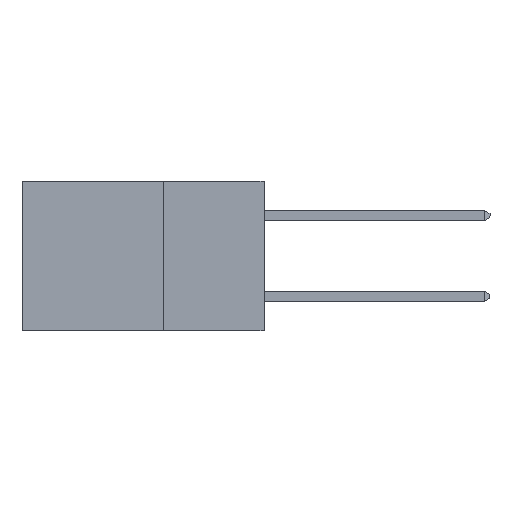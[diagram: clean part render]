
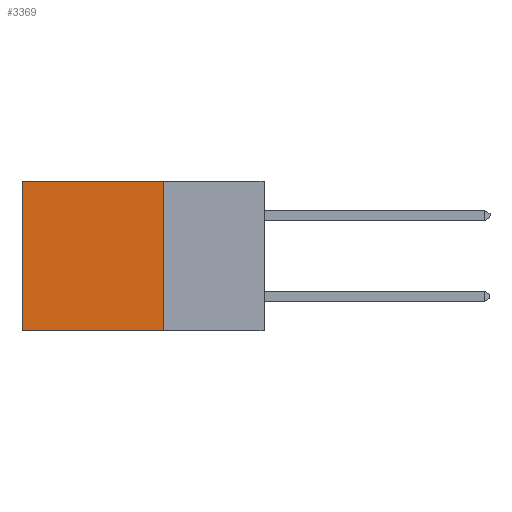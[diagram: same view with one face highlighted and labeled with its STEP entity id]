
A CAD part, left-side view. The second image highlights one B-rep face of the part: STEP entity #3369.
In plain terms, the highlighted planar face has unit normal (-1, 0, 0).
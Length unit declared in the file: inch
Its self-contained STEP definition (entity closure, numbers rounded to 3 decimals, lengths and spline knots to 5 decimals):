
#329 = PLANE ( 'NONE',  #11443 ) ;
#387 = LINE ( 'NONE', #11750, #2366 ) ;
#656 = VERTEX_POINT ( 'NONE', #1639 ) ;
#1639 = CARTESIAN_POINT ( 'NONE',  ( 0.298, 0.6, 0. ) ) ;
#1813 = DIRECTION ( 'NONE',  ( 0., 0., -1. ) ) ;
#2072 = ORIENTED_EDGE ( 'NONE', *, *, #6929, .T. ) ;
#2182 = ORIENTED_EDGE ( 'NONE', *, *, #3774, .F. ) ;
#2245 = VERTEX_POINT ( 'NONE', #4209 ) ;
#2325 = ORIENTED_EDGE ( 'NONE', *, *, #8236, .F. ) ;
#2366 = VECTOR ( 'NONE', #5428, 39.37008 ) ;
#2414 = ORIENTED_EDGE ( 'NONE', *, *, #11624, .T. ) ;
#3369 = ADVANCED_FACE ( 'NONE', ( #8489 ), #329, .F. ) ;
#3519 = DIRECTION ( 'NONE',  ( 1., 0., 0. ) ) ;
#3774 = EDGE_CURVE ( 'NONE', #4103, #2245, #8898, .T. ) ;
#3837 = LINE ( 'NONE', #6218, #11126 ) ;
#4103 = VERTEX_POINT ( 'NONE', #9269 ) ;
#4209 = CARTESIAN_POINT ( 'NONE',  ( 0.298, 0.6, -0.37 ) ) ;
#5428 = DIRECTION ( 'NONE',  ( 0., 0., -1. ) ) ;
#5626 = DIRECTION ( 'NONE',  ( 0., 0., -1. ) ) ;
#6146 = VECTOR ( 'NONE', #5626, 39.37008 ) ;
#6218 = CARTESIAN_POINT ( 'NONE',  ( 0.298, 0.25, 0. ) ) ;
#6403 = VECTOR ( 'NONE', #8607, 39.37008 ) ;
#6642 = CARTESIAN_POINT ( 'NONE',  ( 0.298, 0.25, 0. ) ) ;
#6929 = EDGE_CURVE ( 'NONE', #656, #2245, #10958, .T. ) ;
#7118 = EDGE_LOOP ( 'NONE', ( #2072, #2182, #2325, #2414 ) ) ;
#7720 = VERTEX_POINT ( 'NONE', #9386 ) ;
#8103 = DIRECTION ( 'NONE',  ( 0., 1., 0. ) ) ;
#8236 = EDGE_CURVE ( 'NONE', #7720, #4103, #387, .T. ) ;
#8489 = FACE_OUTER_BOUND ( 'NONE', #7118, .T. ) ;
#8607 = DIRECTION ( 'NONE',  ( 0., 1., 0. ) ) ;
#8772 = CARTESIAN_POINT ( 'NONE',  ( 0.298, 0.25, -0.37 ) ) ;
#8898 = LINE ( 'NONE', #8772, #6403 ) ;
#9269 = CARTESIAN_POINT ( 'NONE',  ( 0.298, 0.25, -0.37 ) ) ;
#9386 = CARTESIAN_POINT ( 'NONE',  ( 0.298, 0.25, 0. ) ) ;
#10958 = LINE ( 'NONE', #11398, #6146 ) ;
#11126 = VECTOR ( 'NONE', #8103, 39.37008 ) ;
#11398 = CARTESIAN_POINT ( 'NONE',  ( 0.298, 0.6, 0. ) ) ;
#11443 = AXIS2_PLACEMENT_3D ( 'NONE', #6642, #3519, #1813 ) ;
#11624 = EDGE_CURVE ( 'NONE', #7720, #656, #3837, .T. ) ;
#11750 = CARTESIAN_POINT ( 'NONE',  ( 0.298, 0.25, 0. ) ) ;
